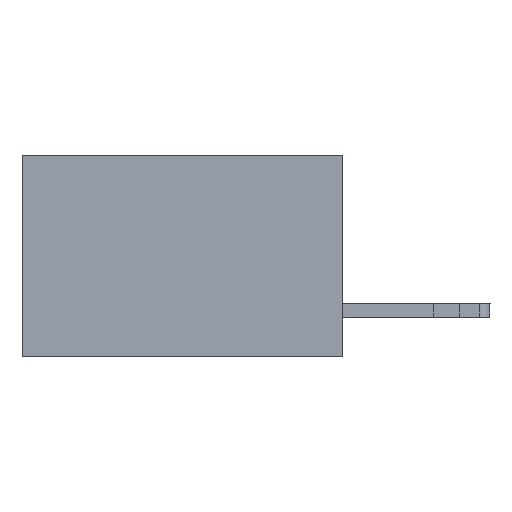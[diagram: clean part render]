
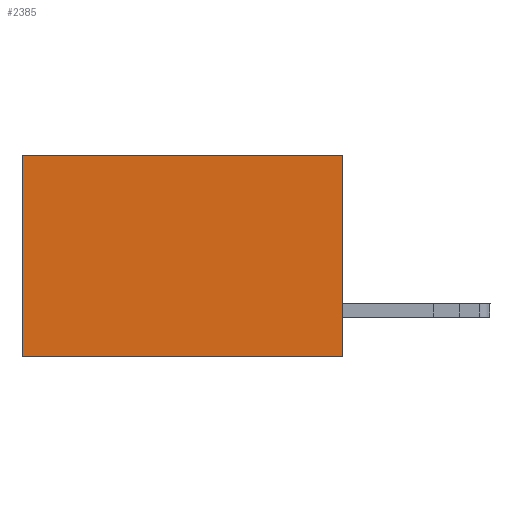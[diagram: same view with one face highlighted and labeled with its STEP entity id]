
A CAD part, left-side view. The second image highlights one B-rep face of the part: STEP entity #2385.
In plain terms, the highlighted planar face has unit normal (-1, 0, 0).
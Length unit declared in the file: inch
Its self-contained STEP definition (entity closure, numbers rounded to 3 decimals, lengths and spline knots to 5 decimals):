
#480 = LINE ( 'NONE', #10945, #10033 ) ;
#2385 = ADVANCED_FACE ( 'NONE', ( #9018 ), #6600, .F. ) ;
#3479 = EDGE_CURVE ( 'NONE', #11831, #10693, #5560, .T. ) ;
#3766 = CARTESIAN_POINT ( 'NONE',  ( 0.277, 0., 0. ) ) ;
#3938 = EDGE_CURVE ( 'NONE', #11831, #14802, #5140, .T. ) ;
#4384 = EDGE_LOOP ( 'NONE', ( #15687, #9508, #9911, #13221 ) ) ;
#4862 = VECTOR ( 'NONE', #6181, 39.37008 ) ;
#4929 = CARTESIAN_POINT ( 'NONE',  ( 0.277, 0., 0. ) ) ;
#5140 = LINE ( 'NONE', #4929, #8166 ) ;
#5197 = VERTEX_POINT ( 'NONE', #11220 ) ;
#5560 = LINE ( 'NONE', #9874, #15192 ) ;
#5837 = CARTESIAN_POINT ( 'NONE',  ( 0.277, 0., -0.37 ) ) ;
#6068 = EDGE_CURVE ( 'NONE', #10693, #5197, #11226, .T. ) ;
#6181 = DIRECTION ( 'NONE',  ( 0., 1., 0. ) ) ;
#6349 = CARTESIAN_POINT ( 'NONE',  ( 0.277, 0., -0.37 ) ) ;
#6542 = DIRECTION ( 'NONE',  ( 1., 0., 0. ) ) ;
#6600 = PLANE ( 'NONE',  #15164 ) ;
#6652 = DIRECTION ( 'NONE',  ( 0., 0., -1. ) ) ;
#8027 = CARTESIAN_POINT ( 'NONE',  ( 0.277, 0., -0.37 ) ) ;
#8166 = VECTOR ( 'NONE', #10262, 39.37008 ) ;
#9018 = FACE_OUTER_BOUND ( 'NONE', #4384, .T. ) ;
#9508 = ORIENTED_EDGE ( 'NONE', *, *, #6068, .F. ) ;
#9874 = CARTESIAN_POINT ( 'NONE',  ( 0.277, 0., -0.37 ) ) ;
#9911 = ORIENTED_EDGE ( 'NONE', *, *, #3479, .F. ) ;
#10033 = VECTOR ( 'NONE', #12184, 39.37008 ) ;
#10199 = DIRECTION ( 'NONE',  ( 0., 0., -1. ) ) ;
#10262 = DIRECTION ( 'NONE',  ( 0., 1., 0. ) ) ;
#10693 = VERTEX_POINT ( 'NONE', #8027 ) ;
#10945 = CARTESIAN_POINT ( 'NONE',  ( 0.277, 0.59, -0.37 ) ) ;
#11220 = CARTESIAN_POINT ( 'NONE',  ( 0.277, 0.59, -0.37 ) ) ;
#11226 = LINE ( 'NONE', #5837, #4862 ) ;
#11831 = VERTEX_POINT ( 'NONE', #3766 ) ;
#12184 = DIRECTION ( 'NONE',  ( 0., 0., -1. ) ) ;
#12915 = CARTESIAN_POINT ( 'NONE',  ( 0.277, 0.59, 0. ) ) ;
#13074 = EDGE_CURVE ( 'NONE', #14802, #5197, #480, .T. ) ;
#13221 = ORIENTED_EDGE ( 'NONE', *, *, #3938, .T. ) ;
#14802 = VERTEX_POINT ( 'NONE', #12915 ) ;
#15164 = AXIS2_PLACEMENT_3D ( 'NONE', #6349, #6542, #6652 ) ;
#15192 = VECTOR ( 'NONE', #10199, 39.37008 ) ;
#15687 = ORIENTED_EDGE ( 'NONE', *, *, #13074, .T. ) ;
